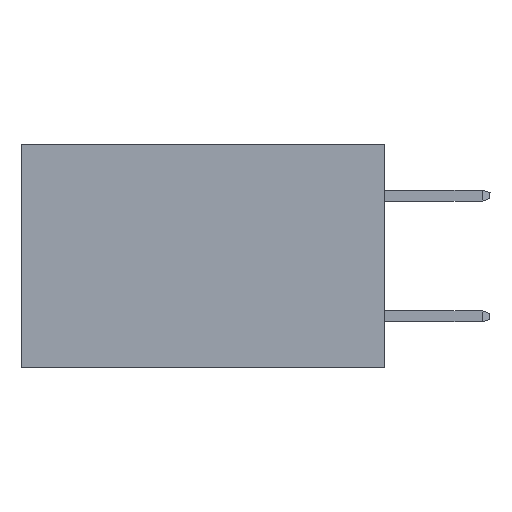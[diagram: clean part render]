
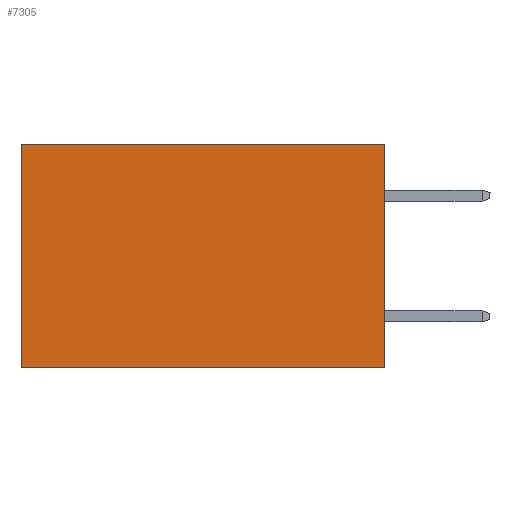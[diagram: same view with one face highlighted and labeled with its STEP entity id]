
A CAD part, left-side view. The second image highlights one B-rep face of the part: STEP entity #7305.
In plain terms, the highlighted planar face has unit normal (-1, 0, 0).
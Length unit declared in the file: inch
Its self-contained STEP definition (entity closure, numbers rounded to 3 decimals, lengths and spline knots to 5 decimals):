
#52 = DIRECTION ( 'NONE',  ( 0., 0., -1. ) ) ;
#170 = EDGE_CURVE ( 'NONE', #10675, #8016, #10739, .T. ) ;
#570 = VERTEX_POINT ( 'NONE', #3787 ) ;
#660 = PLANE ( 'NONE',  #10691 ) ;
#875 = VECTOR ( 'NONE', #52, 39.37008 ) ;
#1141 = CARTESIAN_POINT ( 'NONE',  ( 0.298, 0.6, 0. ) ) ;
#1302 = EDGE_CURVE ( 'NONE', #570, #10675, #1657, .T. ) ;
#1657 = LINE ( 'NONE', #1894, #8300 ) ;
#1894 = CARTESIAN_POINT ( 'NONE',  ( 0.298, 0., 0. ) ) ;
#2421 = VERTEX_POINT ( 'NONE', #9936 ) ;
#2932 = CARTESIAN_POINT ( 'NONE',  ( 0.298, 0.6, 0. ) ) ;
#3330 = CARTESIAN_POINT ( 'NONE',  ( 0.298, 0., 0. ) ) ;
#3355 = ORIENTED_EDGE ( 'NONE', *, *, #1302, .T. ) ;
#3637 = DIRECTION ( 'NONE',  ( 0., 1., 0. ) ) ;
#3739 = ORIENTED_EDGE ( 'NONE', *, *, #4731, .F. ) ;
#3787 = CARTESIAN_POINT ( 'NONE',  ( 0.298, 0., 0. ) ) ;
#4419 = LINE ( 'NONE', #5854, #6738 ) ;
#4731 = EDGE_CURVE ( 'NONE', #2421, #8016, #4419, .T. ) ;
#4981 = DIRECTION ( 'NONE',  ( 1., 0., 0. ) ) ;
#5123 = FACE_OUTER_BOUND ( 'NONE', #6410, .T. ) ;
#5854 = CARTESIAN_POINT ( 'NONE',  ( 0.298, 0., -0.37 ) ) ;
#5960 = DIRECTION ( 'NONE',  ( 0., 1., 0. ) ) ;
#6298 = DIRECTION ( 'NONE',  ( 0., 0., -1. ) ) ;
#6410 = EDGE_LOOP ( 'NONE', ( #8097, #3739, #7500, #3355 ) ) ;
#6738 = VECTOR ( 'NONE', #5960, 39.37008 ) ;
#7305 = ADVANCED_FACE ( 'NONE', ( #5123 ), #660, .F. ) ;
#7500 = ORIENTED_EDGE ( 'NONE', *, *, #9647, .F. ) ;
#7551 = DIRECTION ( 'NONE',  ( 0., 0., -1. ) ) ;
#8016 = VERTEX_POINT ( 'NONE', #9814 ) ;
#8097 = ORIENTED_EDGE ( 'NONE', *, *, #170, .T. ) ;
#8196 = VECTOR ( 'NONE', #6298, 39.37008 ) ;
#8218 = LINE ( 'NONE', #10343, #875 ) ;
#8300 = VECTOR ( 'NONE', #3637, 39.37008 ) ;
#9647 = EDGE_CURVE ( 'NONE', #570, #2421, #8218, .T. ) ;
#9814 = CARTESIAN_POINT ( 'NONE',  ( 0.298, 0.6, -0.37 ) ) ;
#9936 = CARTESIAN_POINT ( 'NONE',  ( 0.298, 0., -0.37 ) ) ;
#10343 = CARTESIAN_POINT ( 'NONE',  ( 0.298, 0., 0. ) ) ;
#10675 = VERTEX_POINT ( 'NONE', #1141 ) ;
#10691 = AXIS2_PLACEMENT_3D ( 'NONE', #3330, #4981, #7551 ) ;
#10739 = LINE ( 'NONE', #2932, #8196 ) ;
